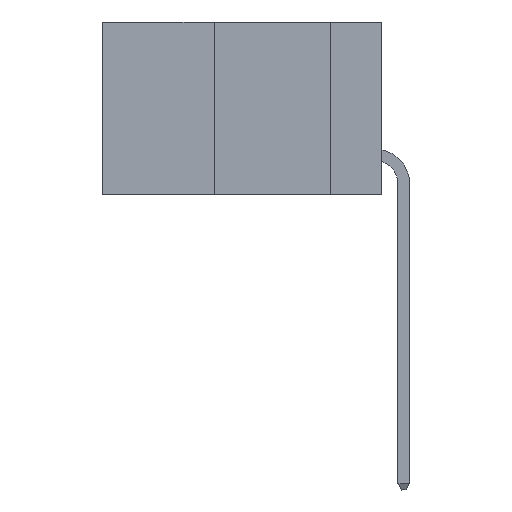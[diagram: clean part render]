
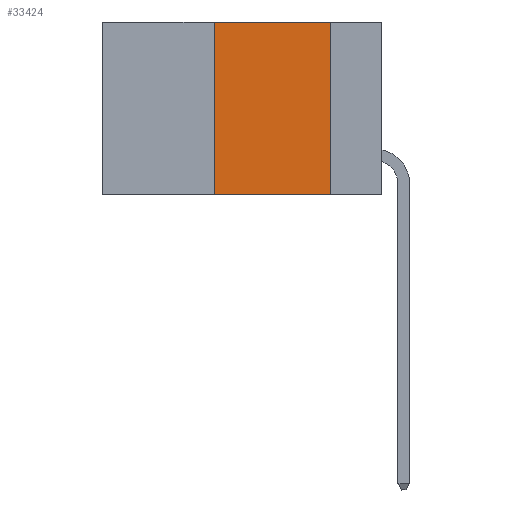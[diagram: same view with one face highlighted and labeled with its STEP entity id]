
A CAD part, left-side view. The second image highlights one B-rep face of the part: STEP entity #33424.
In plain terms, the highlighted planar face has unit normal (-1, 0, 0).
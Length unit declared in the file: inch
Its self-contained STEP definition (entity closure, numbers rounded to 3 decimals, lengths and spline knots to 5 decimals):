
#325 = DIRECTION ( 'NONE',  ( 1., 0., 0. ) ) ;
#351 = VERTEX_POINT ( 'NONE', #34082 ) ;
#3940 = PLANE ( 'NONE',  #13698 ) ;
#4571 = VECTOR ( 'NONE', #16599, 39.37008 ) ;
#6916 = LINE ( 'NONE', #19161, #17561 ) ;
#7420 = CARTESIAN_POINT ( 'NONE',  ( 0., 0.36, 0. ) ) ;
#10043 = ORIENTED_EDGE ( 'NONE', *, *, #29001, .F. ) ;
#10120 = DIRECTION ( 'NONE',  ( 0., 0., -1. ) ) ;
#10727 = CARTESIAN_POINT ( 'NONE',  ( 0., 0.11, 0. ) ) ;
#12057 = VECTOR ( 'NONE', #17986, 39.37008 ) ;
#13698 = AXIS2_PLACEMENT_3D ( 'NONE', #34604, #325, #10120 ) ;
#13863 = ORIENTED_EDGE ( 'NONE', *, *, #15754, .F. ) ;
#15754 = EDGE_CURVE ( 'NONE', #351, #22175, #37046, .T. ) ;
#16368 = ORIENTED_EDGE ( 'NONE', *, *, #28338, .T. ) ;
#16599 = DIRECTION ( 'NONE',  ( 0., -1., 0. ) ) ;
#17455 = CARTESIAN_POINT ( 'NONE',  ( 0., 0.36, 0. ) ) ;
#17561 = VECTOR ( 'NONE', #22247, 39.37008 ) ;
#17986 = DIRECTION ( 'NONE',  ( 0., 0., 1. ) ) ;
#19161 = CARTESIAN_POINT ( 'NONE',  ( 0., 0.6, -0.37 ) ) ;
#20640 = VERTEX_POINT ( 'NONE', #24552 ) ;
#20931 = LINE ( 'NONE', #35006, #4571 ) ;
#22175 = VERTEX_POINT ( 'NONE', #7420 ) ;
#22247 = DIRECTION ( 'NONE',  ( 0., -1., 0. ) ) ;
#22958 = CARTESIAN_POINT ( 'NONE',  ( 0., 0.11, 0. ) ) ;
#24552 = CARTESIAN_POINT ( 'NONE',  ( 0., 0.11, -0.37 ) ) ;
#25872 = DIRECTION ( 'NONE',  ( 0., 0., -1. ) ) ;
#26630 = VECTOR ( 'NONE', #25872, 39.37008 ) ;
#28338 = EDGE_CURVE ( 'NONE', #351, #20640, #6916, .T. ) ;
#29001 = EDGE_CURVE ( 'NONE', #32356, #20640, #39165, .T. ) ;
#30852 = FACE_OUTER_BOUND ( 'NONE', #31847, .T. ) ;
#31105 = EDGE_CURVE ( 'NONE', #22175, #32356, #20931, .T. ) ;
#31847 = EDGE_LOOP ( 'NONE', ( #10043, #37385, #13863, #16368 ) ) ;
#32356 = VERTEX_POINT ( 'NONE', #22958 ) ;
#33424 = ADVANCED_FACE ( 'NONE', ( #30852 ), #3940, .F. ) ;
#34082 = CARTESIAN_POINT ( 'NONE',  ( 0., 0.36, -0.37 ) ) ;
#34604 = CARTESIAN_POINT ( 'NONE',  ( 0., 0.6, 0. ) ) ;
#35006 = CARTESIAN_POINT ( 'NONE',  ( 0., 0.6, 0. ) ) ;
#37046 = LINE ( 'NONE', #17455, #12057 ) ;
#37385 = ORIENTED_EDGE ( 'NONE', *, *, #31105, .F. ) ;
#39165 = LINE ( 'NONE', #10727, #26630 ) ;
